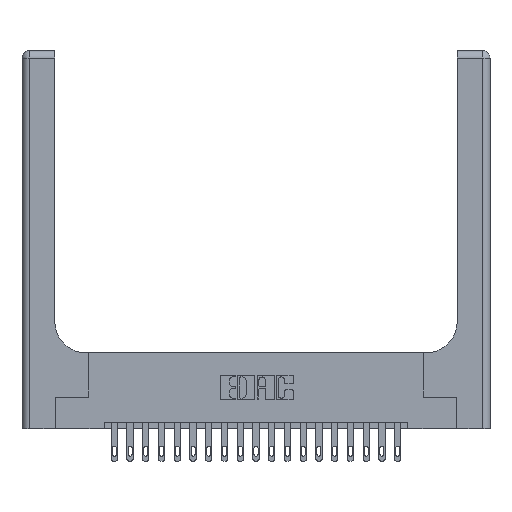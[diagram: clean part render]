
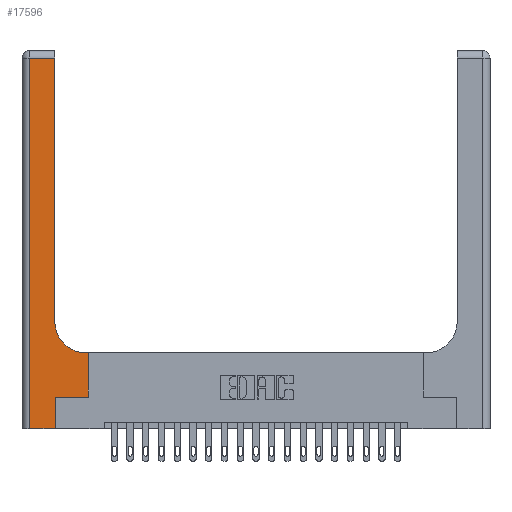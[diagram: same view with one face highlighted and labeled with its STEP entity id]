
A CAD part, top view. The second image highlights one B-rep face of the part: STEP entity #17596.
In plain terms, the highlighted planar face has unit normal (0, 0, 1).
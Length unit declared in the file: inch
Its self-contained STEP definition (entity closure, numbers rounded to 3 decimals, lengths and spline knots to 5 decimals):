
#16 = EDGE_CURVE ( 'NONE', #8573, #17050, #11058, .T. ) ;
#542 = VECTOR ( 'NONE', #19775, 39.37008 ) ;
#622 = VERTEX_POINT ( 'NONE', #18723 ) ;
#740 = EDGE_LOOP ( 'NONE', ( #19088, #6172, #978, #2561, #20887, #3669, #11575, #1339, #5749 ) ) ;
#784 = CARTESIAN_POINT ( 'NONE',  ( 0.51, 0.6, 0.37 ) ) ;
#978 = ORIENTED_EDGE ( 'NONE', *, *, #984, .T. ) ;
#984 = EDGE_CURVE ( 'NONE', #4755, #622, #5382, .T. ) ;
#1339 = ORIENTED_EDGE ( 'NONE', *, *, #16, .T. ) ;
#1494 = FACE_OUTER_BOUND ( 'NONE', #740, .T. ) ;
#1653 = EDGE_CURVE ( 'NONE', #5430, #4755, #20146, .T. ) ;
#2561 = ORIENTED_EDGE ( 'NONE', *, *, #17569, .T. ) ;
#3009 = DIRECTION ( 'NONE',  ( 1., 0., 0. ) ) ;
#3669 = ORIENTED_EDGE ( 'NONE', *, *, #12532, .T. ) ;
#4755 = VERTEX_POINT ( 'NONE', #7493 ) ;
#5382 = LINE ( 'NONE', #13264, #542 ) ;
#5385 = VECTOR ( 'NONE', #9219, 39.37008 ) ;
#5430 = VERTEX_POINT ( 'NONE', #16351 ) ;
#5508 = VECTOR ( 'NONE', #3009, 39.37008 ) ;
#5545 = CARTESIAN_POINT ( 'NONE',  ( 0., 2.94, 0.37 ) ) ;
#5749 = ORIENTED_EDGE ( 'NONE', *, *, #6013, .T. ) ;
#6013 = EDGE_CURVE ( 'NONE', #17050, #11922, #15251, .T. ) ;
#6172 = ORIENTED_EDGE ( 'NONE', *, *, #1653, .T. ) ;
#6197 = VECTOR ( 'NONE', #20096, 39.37008 ) ;
#6233 = LINE ( 'NONE', #10842, #17568 ) ;
#6421 = CARTESIAN_POINT ( 'NONE',  ( 0.528, 0.25, 0.37 ) ) ;
#6737 = CARTESIAN_POINT ( 'NONE',  ( 0.528, 0.6, 0.37 ) ) ;
#7102 = CARTESIAN_POINT ( 'NONE',  ( 0.265, 0., 0.37 ) ) ;
#7308 = VERTEX_POINT ( 'NONE', #12273 ) ;
#7493 = CARTESIAN_POINT ( 'NONE',  ( 0.06, 2.94, 0.37 ) ) ;
#7781 = DIRECTION ( 'NONE',  ( -1., 0., 0. ) ) ;
#7951 = LINE ( 'NONE', #6421, #5385 ) ;
#8106 = PLANE ( 'NONE',  #9213 ) ;
#8114 = VERTEX_POINT ( 'NONE', #11809 ) ;
#8573 = VERTEX_POINT ( 'NONE', #6737 ) ;
#9213 = AXIS2_PLACEMENT_3D ( 'NONE', #14361, #17468, #20884 ) ;
#9219 = DIRECTION ( 'NONE',  ( 0., 1., 0. ) ) ;
#9410 = CARTESIAN_POINT ( 'NONE',  ( 0.26, 3., 0.37 ) ) ;
#9586 = LINE ( 'NONE', #17570, #5508 ) ;
#9587 = EDGE_CURVE ( 'NONE', #10075, #8573, #7951, .T. ) ;
#10075 = VERTEX_POINT ( 'NONE', #14612 ) ;
#10842 = CARTESIAN_POINT ( 'NONE',  ( 0.265, 0.25, 0.37 ) ) ;
#10903 = LINE ( 'NONE', #9410, #15651 ) ;
#11058 = LINE ( 'NONE', #19487, #15092 ) ;
#11575 = ORIENTED_EDGE ( 'NONE', *, *, #9587, .T. ) ;
#11809 = CARTESIAN_POINT ( 'NONE',  ( 0.265, 0., 0.37 ) ) ;
#11922 = VERTEX_POINT ( 'NONE', #15420 ) ;
#12273 = CARTESIAN_POINT ( 'NONE',  ( 0.265, 0.25, 0.37 ) ) ;
#12532 = EDGE_CURVE ( 'NONE', #7308, #10075, #6233, .T. ) ;
#13264 = CARTESIAN_POINT ( 'NONE',  ( 0.06, 3., 0.37 ) ) ;
#13806 = VECTOR ( 'NONE', #7781, 39.37008 ) ;
#14361 = CARTESIAN_POINT ( 'NONE',  ( 0., 3., 0.37 ) ) ;
#14612 = CARTESIAN_POINT ( 'NONE',  ( 0.528, 0.25, 0.37 ) ) ;
#15092 = VECTOR ( 'NONE', #15956, 39.37008 ) ;
#15176 = LINE ( 'NONE', #7102, #6197 ) ;
#15251 = CIRCLE ( 'NONE', #16969, 0.25 ) ;
#15420 = CARTESIAN_POINT ( 'NONE',  ( 0.26, 0.85, 0.37 ) ) ;
#15651 = VECTOR ( 'NONE', #19205, 39.37008 ) ;
#15918 = EDGE_CURVE ( 'NONE', #11922, #5430, #10903, .T. ) ;
#15956 = DIRECTION ( 'NONE',  ( -1., 0., 0. ) ) ;
#16351 = CARTESIAN_POINT ( 'NONE',  ( 0.26, 2.94, 0.37 ) ) ;
#16969 = AXIS2_PLACEMENT_3D ( 'NONE', #18575, #18468, #20571 ) ;
#17050 = VERTEX_POINT ( 'NONE', #784 ) ;
#17329 = DIRECTION ( 'NONE',  ( 1., 0., 0. ) ) ;
#17468 = DIRECTION ( 'NONE',  ( 0., 0., -1. ) ) ;
#17568 = VECTOR ( 'NONE', #17329, 39.37008 ) ;
#17569 = EDGE_CURVE ( 'NONE', #622, #8114, #9586, .T. ) ;
#17570 = CARTESIAN_POINT ( 'NONE',  ( 0., 0., 0.37 ) ) ;
#17596 = ADVANCED_FACE ( 'NONE', ( #1494 ), #8106, .F. ) ;
#18468 = DIRECTION ( 'NONE',  ( 0., 0., -1. ) ) ;
#18575 = CARTESIAN_POINT ( 'NONE',  ( 0.51, 0.85, 0.37 ) ) ;
#18723 = CARTESIAN_POINT ( 'NONE',  ( 0.06, 0., 0.37 ) ) ;
#19088 = ORIENTED_EDGE ( 'NONE', *, *, #15918, .T. ) ;
#19205 = DIRECTION ( 'NONE',  ( 0., 1., 0. ) ) ;
#19487 = CARTESIAN_POINT ( 'NONE',  ( 0.26, 0.6, 0.37 ) ) ;
#19775 = DIRECTION ( 'NONE',  ( 0., -1., 0. ) ) ;
#19779 = EDGE_CURVE ( 'NONE', #8114, #7308, #15176, .T. ) ;
#20096 = DIRECTION ( 'NONE',  ( 0., 1., 0. ) ) ;
#20146 = LINE ( 'NONE', #5545, #13806 ) ;
#20571 = DIRECTION ( 'NONE',  ( 1., 0., 0. ) ) ;
#20884 = DIRECTION ( 'NONE',  ( -1., 0., 0. ) ) ;
#20887 = ORIENTED_EDGE ( 'NONE', *, *, #19779, .T. ) ;
